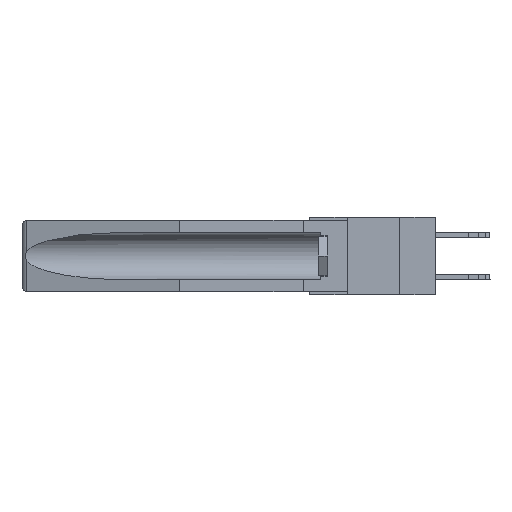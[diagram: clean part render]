
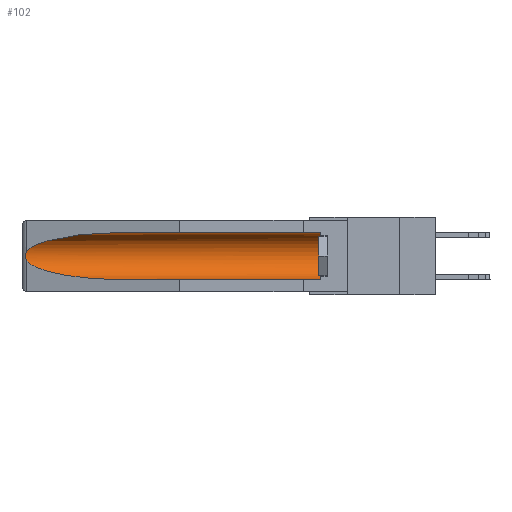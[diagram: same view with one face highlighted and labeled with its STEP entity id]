
A CAD part, left-side view. The second image highlights one B-rep face of the part: STEP entity #102.
In plain terms, the highlighted cylindrical face has radius 2.857 mm (diameter 5.715 mm), a partial arc.
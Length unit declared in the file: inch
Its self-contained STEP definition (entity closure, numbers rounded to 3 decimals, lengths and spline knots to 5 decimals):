
#63 = CARTESIAN_POINT ( 'NONE',  ( 0.26597, 1.52961, -0.15275 ) ) ;
#102 = ADVANCED_FACE ( 'NONE', ( #16993 ), #2406, .F. ) ;
#367 = CARTESIAN_POINT ( 'NONE',  ( 0.26537, 1.52718, -0.19328 ) ) ;
#691 = ORIENTED_EDGE ( 'NONE', *, *, #10334, .T. ) ;
#719 = VERTEX_POINT ( 'NONE', #10195 ) ;
#1292 = CARTESIAN_POINT ( 'NONE',  ( 0.26597, 1.5296, -0.19026 ) ) ;
#1377 = EDGE_CURVE ( 'NONE', #3864, #5209, #16889, .T. ) ;
#1394 = CARTESIAN_POINT ( 'NONE',  ( 0.155, -0.30754, -0.1715 ) ) ;
#2028 = CARTESIAN_POINT ( 'NONE',  ( 0.155, -0.30754, -0.059 ) ) ;
#2406 = CYLINDRICAL_SURFACE ( 'NONE', #7682, 0.1125 ) ;
#3051 = DIRECTION ( 'NONE',  ( 0., 1., 0. ) ) ;
#3864 = VERTEX_POINT ( 'NONE', #16955 ) ;
#4057 = CARTESIAN_POINT ( 'NONE',  ( 0.2675, 1.53308, -0.17534 ) ) ;
#4281 = VERTEX_POINT ( 'NONE', #16919 ) ;
#4591 = CIRCLE ( 'NONE', #8014, 0.1125 ) ;
#4715 = CARTESIAN_POINT ( 'NONE',  ( 0.26537, 1.52718, -0.14972 ) ) ;
#4868 = B_SPLINE_CURVE_WITH_KNOTS ( 'NONE', 3,
 ( #7050, #63, #9773, #18152, #9649, #4057, #13906, #11191, #1292, #5467 ),
 .UNSPECIFIED., .F., .F.,
 ( 4, 2, 2, 2, 4 ),
 ( 0., 0.00029, 0.00058, 0.00087, 0.00117 ),
 .UNSPECIFIED. ) ;
#4886 = DIRECTION ( 'NONE',  ( 0., 0., 1. ) ) ;
#5209 = VERTEX_POINT ( 'NONE', #9347 ) ;
#5325 = ORIENTED_EDGE ( 'NONE', *, *, #7601, .T. ) ;
#5467 = CARTESIAN_POINT ( 'NONE',  ( 0.26537, 1.52718, -0.19328 ) ) ;
#5778 = VERTEX_POINT ( 'NONE', #13101 ) ;
#6295 = VECTOR ( 'NONE', #7679, 39.37008 ) ;
#7050 = CARTESIAN_POINT ( 'NONE',  ( 0.26537, 1.52718, -0.14972 ) ) ;
#7283 = CARTESIAN_POINT ( 'NONE',  ( 0.155, 0.126, -0.1715 ) ) ;
#7475 = DIRECTION ( 'NONE',  ( 0., -1., 0. ) ) ;
#7595 = VERTEX_POINT ( 'NONE', #4715 ) ;
#7601 = EDGE_CURVE ( 'NONE', #4281, #5778, #4591, .T. ) ;
#7632 = ORIENTED_EDGE ( 'NONE', *, *, #11601, .T. ) ;
#7679 = DIRECTION ( 'NONE',  ( 0., 1., 0. ) ) ;
#7682 = AXIS2_PLACEMENT_3D ( 'NONE', #1394, #3051, #16932 ) ;
#8014 = AXIS2_PLACEMENT_3D ( 'NONE', #7283, #7475, #4886 ) ;
#9106 = ORIENTED_EDGE ( 'NONE', *, *, #9713, .F. ) ;
#9347 = CARTESIAN_POINT ( 'NONE',  ( 0.155, 1.07973, -0.284 ) ) ;
#9415 = LINE ( 'NONE', #2028, #6295 ) ;
#9649 = CARTESIAN_POINT ( 'NONE',  ( 0.2675, 1.53308, -0.16763 ) ) ;
#9713 = EDGE_CURVE ( 'NONE', #4281, #5209, #17666, .T. ) ;
#9773 = CARTESIAN_POINT ( 'NONE',  ( 0.26654, 1.53092, -0.15636 ) ) ;
#9916 = CARTESIAN_POINT ( 'NONE',  ( 0.26537, 1.52718, -0.14972 ) ) ;
#10139 = CARTESIAN_POINT ( 'NONE',  ( 0.25451, 1.48313, -0.24835 ) ) ;
#10195 = CARTESIAN_POINT ( 'NONE',  ( 0.155, 1.07973, -0.059 ) ) ;
#10334 = EDGE_CURVE ( 'NONE', #719, #7595, #16649, .T. ) ;
#10529 = ORIENTED_EDGE ( 'NONE', *, *, #1377, .T. ) ;
#11191 = CARTESIAN_POINT ( 'NONE',  ( 0.26655, 1.53094, -0.18657 ) ) ;
#11601 = EDGE_CURVE ( 'NONE', #5778, #719, #9415, .T. ) ;
#11634 = CARTESIAN_POINT ( 'NONE',  ( 0.21114, 1.30732, -0.284 ) ) ;
#12780 = CARTESIAN_POINT ( 'NONE',  ( 0.155, -0.30754, -0.284 ) ) ;
#13070 = EDGE_CURVE ( 'NONE', #7595, #3864, #4868, .T. ) ;
#13101 = CARTESIAN_POINT ( 'NONE',  ( 0.155, 0.126, -0.059 ) ) ;
#13906 = CARTESIAN_POINT ( 'NONE',  ( 0.2673, 1.53269, -0.17917 ) ) ;
#14100 = CARTESIAN_POINT ( 'NONE',  ( 0.25451, 1.48313, -0.09465 ) ) ;
#14176 = DIRECTION ( 'NONE',  ( 0., 1., 0. ) ) ;
#15036 = ORIENTED_EDGE ( 'NONE', *, *, #13070, .T. ) ;
#15484 = CARTESIAN_POINT ( 'NONE',  ( 0.155, 1.07973, -0.059 ) ) ;
#15669 = CARTESIAN_POINT ( 'NONE',  ( 0.21114, 1.30732, -0.059 ) ) ;
#16649 =( BOUNDED_CURVE ( )  B_SPLINE_CURVE ( 3, ( #15484, #15669, #14100, #9916 ),
 .UNSPECIFIED., .F., .F. ) 
 B_SPLINE_CURVE_WITH_KNOTS ( ( 4, 4 ),
 ( 4.71239, 6.08839 ),
 .UNSPECIFIED. ) 
 CURVE ( )  GEOMETRIC_REPRESENTATION_ITEM ( )  RATIONAL_B_SPLINE_CURVE ( ( 1., 0.848, 0.848, 1. ) ) 
 REPRESENTATION_ITEM ( '' )  );
#16889 =( BOUNDED_CURVE ( )  B_SPLINE_CURVE ( 3, ( #367, #10139, #11634, #17207 ),
 .UNSPECIFIED., .F., .F. ) 
 B_SPLINE_CURVE_WITH_KNOTS ( ( 4, 4 ),
 ( 0.1948, 1.5708 ),
 .UNSPECIFIED. ) 
 CURVE ( )  GEOMETRIC_REPRESENTATION_ITEM ( )  RATIONAL_B_SPLINE_CURVE ( ( 1., 0.848, 0.848, 1. ) ) 
 REPRESENTATION_ITEM ( '' )  );
#16919 = CARTESIAN_POINT ( 'NONE',  ( 0.155, 0.126, -0.284 ) ) ;
#16932 = DIRECTION ( 'NONE',  ( 0., 0., 1. ) ) ;
#16955 = CARTESIAN_POINT ( 'NONE',  ( 0.26537, 1.52718, -0.19328 ) ) ;
#16993 = FACE_OUTER_BOUND ( 'NONE', #17506, .T. ) ;
#16998 = VECTOR ( 'NONE', #14176, 39.37008 ) ;
#17207 = CARTESIAN_POINT ( 'NONE',  ( 0.155, 1.07973, -0.284 ) ) ;
#17506 = EDGE_LOOP ( 'NONE', ( #691, #15036, #10529, #9106, #5325, #7632 ) ) ;
#17666 = LINE ( 'NONE', #12780, #16998 ) ;
#18152 = CARTESIAN_POINT ( 'NONE',  ( 0.2673, 1.5327, -0.16383 ) ) ;
